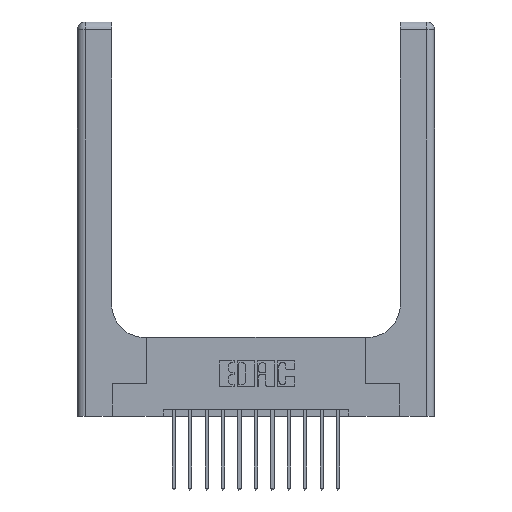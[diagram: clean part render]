
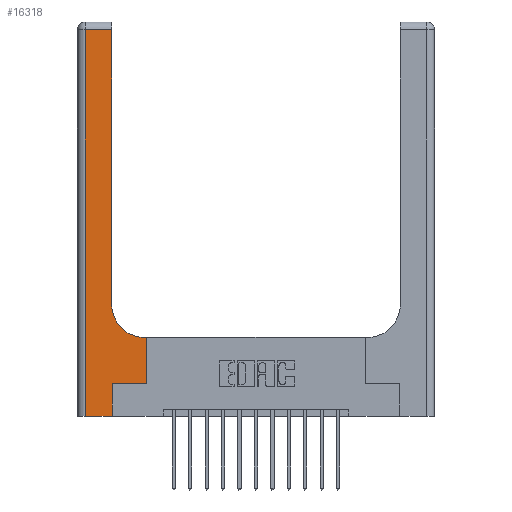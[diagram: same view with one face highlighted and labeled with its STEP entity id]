
A CAD part, top view. The second image highlights one B-rep face of the part: STEP entity #16318.
In plain terms, the highlighted planar face has unit normal (0, 0, 1).
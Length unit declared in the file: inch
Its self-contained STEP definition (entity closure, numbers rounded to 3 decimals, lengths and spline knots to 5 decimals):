
#121 = VERTEX_POINT ( 'NONE', #10106 ) ;
#256 = CARTESIAN_POINT ( 'NONE',  ( 0., 3., 0.37 ) ) ;
#295 = ORIENTED_EDGE ( 'NONE', *, *, #4024, .T. ) ;
#314 = DIRECTION ( 'NONE',  ( 0., 1., 0. ) ) ;
#556 = CARTESIAN_POINT ( 'NONE',  ( 0.06, 3., 0.37 ) ) ;
#1150 = EDGE_CURVE ( 'NONE', #121, #10672, #13193, .T. ) ;
#1199 = LINE ( 'NONE', #11703, #3911 ) ;
#1433 = DIRECTION ( 'NONE',  ( -1., 0., 0. ) ) ;
#1723 = DIRECTION ( 'NONE',  ( 1., 0., 0. ) ) ;
#1814 = EDGE_LOOP ( 'NONE', ( #295, #10725, #4151, #9237, #15063, #2350, #7659, #15416, #14623 ) ) ;
#2156 = CARTESIAN_POINT ( 'NONE',  ( 0.26, 2.94, 0.37 ) ) ;
#2350 = ORIENTED_EDGE ( 'NONE', *, *, #11313, .T. ) ;
#2597 = CARTESIAN_POINT ( 'NONE',  ( 0.26, 0.6, 0.37 ) ) ;
#2881 = VECTOR ( 'NONE', #1723, 39.37008 ) ;
#2926 = DIRECTION ( 'NONE',  ( -1., 0., 0. ) ) ;
#3037 = CARTESIAN_POINT ( 'NONE',  ( 0.528, 0.6, 0.37 ) ) ;
#3282 = EDGE_CURVE ( 'NONE', #10138, #8960, #1199, .T. ) ;
#3539 = EDGE_CURVE ( 'NONE', #13990, #11305, #12299, .T. ) ;
#3550 = DIRECTION ( 'NONE',  ( 1., 0., 0. ) ) ;
#3643 = DIRECTION ( 'NONE',  ( 0., 1., 0. ) ) ;
#3706 = VECTOR ( 'NONE', #5872, 39.37008 ) ;
#3817 = VERTEX_POINT ( 'NONE', #10208 ) ;
#3896 = LINE ( 'NONE', #2597, #14253 ) ;
#3911 = VECTOR ( 'NONE', #3550, 39.37008 ) ;
#4024 = EDGE_CURVE ( 'NONE', #10672, #4452, #6522, .T. ) ;
#4151 = ORIENTED_EDGE ( 'NONE', *, *, #13254, .T. ) ;
#4230 = VERTEX_POINT ( 'NONE', #6753 ) ;
#4452 = VERTEX_POINT ( 'NONE', #2156 ) ;
#4757 = CARTESIAN_POINT ( 'NONE',  ( 0.51, 0.85, 0.37 ) ) ;
#5209 = EDGE_CURVE ( 'NONE', #11305, #121, #3896, .T. ) ;
#5524 = PLANE ( 'NONE',  #7062 ) ;
#5718 = LINE ( 'NONE', #14871, #7571 ) ;
#5819 = CARTESIAN_POINT ( 'NONE',  ( 0.528, 0.25, 0.37 ) ) ;
#5872 = DIRECTION ( 'NONE',  ( 0., 1., 0. ) ) ;
#6522 = LINE ( 'NONE', #11745, #16429 ) ;
#6753 = CARTESIAN_POINT ( 'NONE',  ( 0.06, 2.94, 0.37 ) ) ;
#7034 = LINE ( 'NONE', #556, #8616 ) ;
#7062 = AXIS2_PLACEMENT_3D ( 'NONE', #256, #9546, #1433 ) ;
#7571 = VECTOR ( 'NONE', #2926, 39.37008 ) ;
#7659 = ORIENTED_EDGE ( 'NONE', *, *, #3539, .T. ) ;
#7715 = EDGE_CURVE ( 'NONE', #8960, #3817, #13011, .T. ) ;
#8008 = AXIS2_PLACEMENT_3D ( 'NONE', #4757, #13834, #13912 ) ;
#8184 = FACE_OUTER_BOUND ( 'NONE', #1814, .T. ) ;
#8305 = CARTESIAN_POINT ( 'NONE',  ( 0.265, 0.25, 0.37 ) ) ;
#8408 = CARTESIAN_POINT ( 'NONE',  ( 0.265, 0., 0.37 ) ) ;
#8616 = VECTOR ( 'NONE', #12255, 39.37008 ) ;
#8960 = VERTEX_POINT ( 'NONE', #8408 ) ;
#9073 = EDGE_CURVE ( 'NONE', #4452, #4230, #5718, .T. ) ;
#9237 = ORIENTED_EDGE ( 'NONE', *, *, #3282, .T. ) ;
#9546 = DIRECTION ( 'NONE',  ( 0., 0., -1. ) ) ;
#10106 = CARTESIAN_POINT ( 'NONE',  ( 0.51, 0.6, 0.37 ) ) ;
#10138 = VERTEX_POINT ( 'NONE', #15703 ) ;
#10208 = CARTESIAN_POINT ( 'NONE',  ( 0.265, 0.25, 0.37 ) ) ;
#10672 = VERTEX_POINT ( 'NONE', #12819 ) ;
#10725 = ORIENTED_EDGE ( 'NONE', *, *, #9073, .T. ) ;
#11061 = CARTESIAN_POINT ( 'NONE',  ( 0.528, 0.25, 0.37 ) ) ;
#11305 = VERTEX_POINT ( 'NONE', #3037 ) ;
#11313 = EDGE_CURVE ( 'NONE', #3817, #13990, #16201, .T. ) ;
#11537 = DIRECTION ( 'NONE',  ( -1., 0., 0. ) ) ;
#11703 = CARTESIAN_POINT ( 'NONE',  ( 0., 0., 0.37 ) ) ;
#11713 = CARTESIAN_POINT ( 'NONE',  ( 0.265, 0., 0.37 ) ) ;
#11745 = CARTESIAN_POINT ( 'NONE',  ( 0.26, 3., 0.37 ) ) ;
#12255 = DIRECTION ( 'NONE',  ( 0., -1., 0. ) ) ;
#12299 = LINE ( 'NONE', #11061, #3706 ) ;
#12819 = CARTESIAN_POINT ( 'NONE',  ( 0.26, 0.85, 0.37 ) ) ;
#13011 = LINE ( 'NONE', #11713, #15476 ) ;
#13193 = CIRCLE ( 'NONE', #8008, 0.25 ) ;
#13254 = EDGE_CURVE ( 'NONE', #4230, #10138, #7034, .T. ) ;
#13834 = DIRECTION ( 'NONE',  ( 0., 0., -1. ) ) ;
#13912 = DIRECTION ( 'NONE',  ( 1., 0., 0. ) ) ;
#13990 = VERTEX_POINT ( 'NONE', #5819 ) ;
#14253 = VECTOR ( 'NONE', #11537, 39.37008 ) ;
#14623 = ORIENTED_EDGE ( 'NONE', *, *, #1150, .T. ) ;
#14871 = CARTESIAN_POINT ( 'NONE',  ( 0., 2.94, 0.37 ) ) ;
#15063 = ORIENTED_EDGE ( 'NONE', *, *, #7715, .T. ) ;
#15416 = ORIENTED_EDGE ( 'NONE', *, *, #5209, .T. ) ;
#15476 = VECTOR ( 'NONE', #3643, 39.37008 ) ;
#15703 = CARTESIAN_POINT ( 'NONE',  ( 0.06, 0., 0.37 ) ) ;
#16201 = LINE ( 'NONE', #8305, #2881 ) ;
#16318 = ADVANCED_FACE ( 'NONE', ( #8184 ), #5524, .F. ) ;
#16429 = VECTOR ( 'NONE', #314, 39.37008 ) ;
